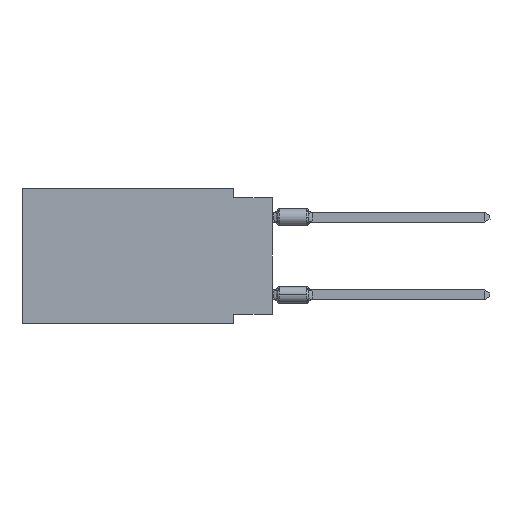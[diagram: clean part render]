
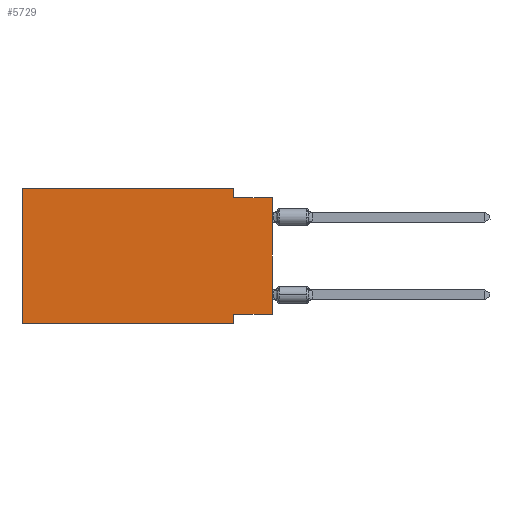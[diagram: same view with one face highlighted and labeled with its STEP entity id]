
A CAD part, left-side view. The second image highlights one B-rep face of the part: STEP entity #5729.
In plain terms, the highlighted planar face has unit normal (-1, 0, 0).
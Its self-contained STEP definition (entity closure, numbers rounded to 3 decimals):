
#541 = LINE ( 'NONE', #2370, #16043 ) ;
#728 = VERTEX_POINT ( 'NONE', #18119 ) ;
#760 = CARTESIAN_POINT ( 'NONE',  ( 0., 16.383, 0. ) ) ;
#878 = EDGE_CURVE ( 'NONE', #22526, #16784, #12888, .T. ) ;
#1092 = ORIENTED_EDGE ( 'NONE', *, *, #14546, .F. ) ;
#1171 = ORIENTED_EDGE ( 'NONE', *, *, #19794, .F. ) ;
#2370 = CARTESIAN_POINT ( 'NONE',  ( 0., 2.54, 0. ) ) ;
#3031 = LINE ( 'NONE', #9933, #19323 ) ;
#4103 = ORIENTED_EDGE ( 'NONE', *, *, #8539, .F. ) ;
#4325 = DIRECTION ( 'NONE',  ( 0., -1., 0. ) ) ;
#4853 = VECTOR ( 'NONE', #18451, 1000. ) ;
#5193 = ORIENTED_EDGE ( 'NONE', *, *, #18588, .F. ) ;
#5380 = CARTESIAN_POINT ( 'NONE',  ( 0., 2.54, -8.89 ) ) ;
#5493 = PLANE ( 'NONE',  #13227 ) ;
#5641 = CARTESIAN_POINT ( 'NONE',  ( 0., 2.54, -8.255 ) ) ;
#5702 = LINE ( 'NONE', #20079, #14270 ) ;
#5729 = ADVANCED_FACE ( 'NONE', ( #13905 ), #5493, .F. ) ;
#6023 = LINE ( 'NONE', #7753, #8660 ) ;
#7414 = VECTOR ( 'NONE', #22053, 1000. ) ;
#7753 = CARTESIAN_POINT ( 'NONE',  ( 0., 0., -0.635 ) ) ;
#8106 = LINE ( 'NONE', #9589, #4853 ) ;
#8499 = CARTESIAN_POINT ( 'NONE',  ( 0., 16.383, 0. ) ) ;
#8514 = EDGE_CURVE ( 'NONE', #18818, #9524, #8106, .T. ) ;
#8539 = EDGE_CURVE ( 'NONE', #22526, #12914, #16717, .T. ) ;
#8660 = VECTOR ( 'NONE', #21809, 1000. ) ;
#8981 = ORIENTED_EDGE ( 'NONE', *, *, #878, .T. ) ;
#9524 = VERTEX_POINT ( 'NONE', #17916 ) ;
#9551 = EDGE_LOOP ( 'NONE', ( #14742, #19859, #19026, #5193, #4103, #8981, #1171, #1092 ) ) ;
#9589 = CARTESIAN_POINT ( 'NONE',  ( 0., 0., 0. ) ) ;
#9933 = CARTESIAN_POINT ( 'NONE',  ( 0., 0., -8.255 ) ) ;
#9972 = DIRECTION ( 'NONE',  ( 0., 0., -1. ) ) ;
#11593 = LINE ( 'NONE', #18597, #12116 ) ;
#11645 = CARTESIAN_POINT ( 'NONE',  ( 0., 16.383, -8.89 ) ) ;
#11784 = DIRECTION ( 'NONE',  ( 0., 1., 0. ) ) ;
#12116 = VECTOR ( 'NONE', #9972, 1000. ) ;
#12888 = LINE ( 'NONE', #14277, #21551 ) ;
#12914 = VERTEX_POINT ( 'NONE', #13413 ) ;
#13227 = AXIS2_PLACEMENT_3D ( 'NONE', #8499, #20813, #17796 ) ;
#13413 = CARTESIAN_POINT ( 'NONE',  ( 0., 16.383, 0. ) ) ;
#13905 = FACE_OUTER_BOUND ( 'NONE', #9551, .T. ) ;
#14270 = VECTOR ( 'NONE', #4325, 1000. ) ;
#14277 = CARTESIAN_POINT ( 'NONE',  ( 0., 16.383, -8.89 ) ) ;
#14546 = EDGE_CURVE ( 'NONE', #18818, #15894, #3031, .T. ) ;
#14742 = ORIENTED_EDGE ( 'NONE', *, *, #8514, .T. ) ;
#15604 = EDGE_CURVE ( 'NONE', #21681, #9524, #6023, .T. ) ;
#15682 = CARTESIAN_POINT ( 'NONE',  ( 0., 0., -8.255 ) ) ;
#15894 = VERTEX_POINT ( 'NONE', #5641 ) ;
#16043 = VECTOR ( 'NONE', #21256, 1000. ) ;
#16717 = LINE ( 'NONE', #760, #7414 ) ;
#16784 = VERTEX_POINT ( 'NONE', #5380 ) ;
#17252 = EDGE_CURVE ( 'NONE', #728, #21681, #541, .T. ) ;
#17796 = DIRECTION ( 'NONE',  ( 0., 0., -1. ) ) ;
#17916 = CARTESIAN_POINT ( 'NONE',  ( 0., 0., -0.635 ) ) ;
#18119 = CARTESIAN_POINT ( 'NONE',  ( 0., 2.54, 0. ) ) ;
#18451 = DIRECTION ( 'NONE',  ( 0., 0., 1. ) ) ;
#18588 = EDGE_CURVE ( 'NONE', #12914, #728, #5702, .T. ) ;
#18597 = CARTESIAN_POINT ( 'NONE',  ( 0., 2.54, -8.89 ) ) ;
#18818 = VERTEX_POINT ( 'NONE', #15682 ) ;
#19026 = ORIENTED_EDGE ( 'NONE', *, *, #17252, .F. ) ;
#19323 = VECTOR ( 'NONE', #11784, 1000. ) ;
#19794 = EDGE_CURVE ( 'NONE', #15894, #16784, #11593, .T. ) ;
#19859 = ORIENTED_EDGE ( 'NONE', *, *, #15604, .F. ) ;
#20079 = CARTESIAN_POINT ( 'NONE',  ( 0., 16.383, 0. ) ) ;
#20813 = DIRECTION ( 'NONE',  ( 1., 0., 0. ) ) ;
#21191 = DIRECTION ( 'NONE',  ( 0., -1., 0. ) ) ;
#21256 = DIRECTION ( 'NONE',  ( 0., 0., -1. ) ) ;
#21551 = VECTOR ( 'NONE', #21191, 1000. ) ;
#21681 = VERTEX_POINT ( 'NONE', #22306 ) ;
#21809 = DIRECTION ( 'NONE',  ( 0., -1., 0. ) ) ;
#22053 = DIRECTION ( 'NONE',  ( 0., 0., 1. ) ) ;
#22306 = CARTESIAN_POINT ( 'NONE',  ( 0., 2.54, -0.635 ) ) ;
#22526 = VERTEX_POINT ( 'NONE', #11645 ) ;
